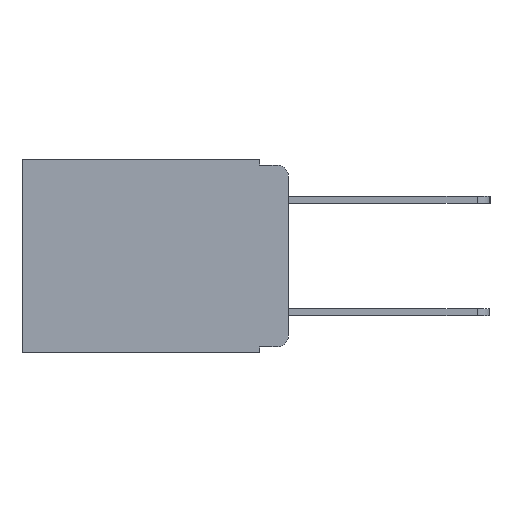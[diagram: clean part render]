
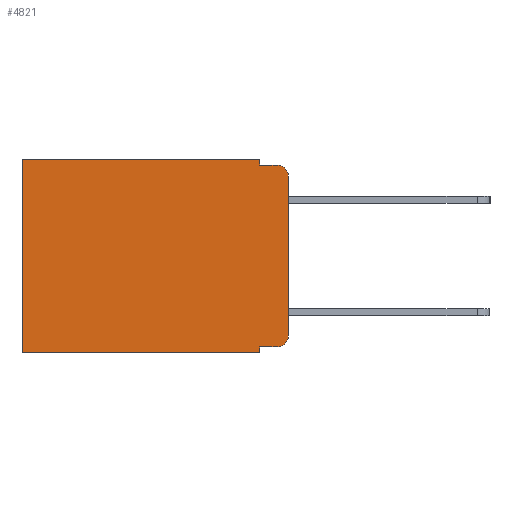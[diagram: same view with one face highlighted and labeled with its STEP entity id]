
A CAD part, left-side view. The second image highlights one B-rep face of the part: STEP entity #4821.
In plain terms, the highlighted planar face has unit normal (-1, 0, 0).
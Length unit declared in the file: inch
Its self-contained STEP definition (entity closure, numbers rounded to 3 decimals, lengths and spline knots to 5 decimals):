
#98 = DIRECTION ( 'NONE',  ( 0., 1., 0. ) ) ;
#150 = CARTESIAN_POINT ( 'NONE',  ( 0.298, 0.473, -0.343 ) ) ;
#318 = ORIENTED_EDGE ( 'NONE', *, *, #4238, .F. ) ;
#379 = VERTEX_POINT ( 'NONE', #12197 ) ;
#389 = PLANE ( 'NONE',  #3781 ) ;
#594 = DIRECTION ( 'NONE',  ( 0., 0., -1. ) ) ;
#773 = ORIENTED_EDGE ( 'NONE', *, *, #3986, .F. ) ;
#1186 = VECTOR ( 'NONE', #10258, 39.37008 ) ;
#1229 = ORIENTED_EDGE ( 'NONE', *, *, #4241, .T. ) ;
#1280 = CARTESIAN_POINT ( 'NONE',  ( 0.298, 0., -0.343 ) ) ;
#1555 = ORIENTED_EDGE ( 'NONE', *, *, #4210, .F. ) ;
#1888 = DIRECTION ( 'NONE',  ( -1., 0., 0. ) ) ;
#2179 = LINE ( 'NONE', #10203, #5570 ) ;
#2844 = DIRECTION ( 'NONE',  ( 0., 1., 0. ) ) ;
#2897 = CARTESIAN_POINT ( 'NONE',  ( 0.298, 0.051, -0.333 ) ) ;
#3305 = DIRECTION ( 'NONE',  ( 0., 0., -1. ) ) ;
#3537 = CARTESIAN_POINT ( 'NONE',  ( 0.298, 0., 0. ) ) ;
#3640 = EDGE_CURVE ( 'NONE', #8289, #14231, #14062, .T. ) ;
#3781 = AXIS2_PLACEMENT_3D ( 'NONE', #3537, #12635, #4957 ) ;
#3828 = CARTESIAN_POINT ( 'NONE',  ( 0.298, 0., -0.313 ) ) ;
#3986 = EDGE_CURVE ( 'NONE', #13887, #12372, #10531, .T. ) ;
#4166 = EDGE_CURVE ( 'NONE', #379, #12834, #6839, .T. ) ;
#4185 = EDGE_CURVE ( 'NONE', #379, #5580, #13086, .T. ) ;
#4210 = EDGE_CURVE ( 'NONE', #14830, #5580, #9556, .T. ) ;
#4213 = EDGE_CURVE ( 'NONE', #8289, #14830, #2179, .T. ) ;
#4215 = EDGE_CURVE ( 'NONE', #14231, #12372, #9168, .T. ) ;
#4238 = EDGE_CURVE ( 'NONE', #14601, #13887, #5143, .T. ) ;
#4241 = EDGE_CURVE ( 'NONE', #14601, #8076, #12006, .T. ) ;
#4269 = EDGE_CURVE ( 'NONE', #8076, #12834, #8367, .T. ) ;
#4493 = AXIS2_PLACEMENT_3D ( 'NONE', #10161, #1888, #11385 ) ;
#4821 = ADVANCED_FACE ( 'NONE', ( #11829 ), #389, .F. ) ;
#4917 = DIRECTION ( 'NONE',  ( 0., 0., -1. ) ) ;
#4957 = DIRECTION ( 'NONE',  ( 0., 0., -1. ) ) ;
#5143 = LINE ( 'NONE', #14980, #1186 ) ;
#5570 = VECTOR ( 'NONE', #4917, 39.37008 ) ;
#5580 = VERTEX_POINT ( 'NONE', #13202 ) ;
#5706 = ORIENTED_EDGE ( 'NONE', *, *, #4215, .T. ) ;
#6314 = CARTESIAN_POINT ( 'NONE',  ( 0.298, 0.051, -0.333 ) ) ;
#6353 = CARTESIAN_POINT ( 'NONE',  ( 0.298, 0.051, -0.01 ) ) ;
#6839 = LINE ( 'NONE', #10111, #9954 ) ;
#7806 = ORIENTED_EDGE ( 'NONE', *, *, #4166, .F. ) ;
#8076 = VERTEX_POINT ( 'NONE', #8678 ) ;
#8214 = ORIENTED_EDGE ( 'NONE', *, *, #4269, .T. ) ;
#8289 = VERTEX_POINT ( 'NONE', #11605 ) ;
#8367 = CIRCLE ( 'NONE', #10673, 0.02 ) ;
#8422 = ORIENTED_EDGE ( 'NONE', *, *, #4185, .T. ) ;
#8613 = ORIENTED_EDGE ( 'NONE', *, *, #4213, .F. ) ;
#8678 = CARTESIAN_POINT ( 'NONE',  ( 0.298, 0.02, -0.333 ) ) ;
#9118 = ORIENTED_EDGE ( 'NONE', *, *, #3640, .T. ) ;
#9121 = DIRECTION ( 'NONE',  ( -1., 0., 0. ) ) ;
#9168 = LINE ( 'NONE', #14935, #15105 ) ;
#9556 = LINE ( 'NONE', #11443, #12366 ) ;
#9954 = VECTOR ( 'NONE', #3305, 39.37008 ) ;
#9975 = CARTESIAN_POINT ( 'NONE',  ( 0.298, 0., 0. ) ) ;
#10111 = CARTESIAN_POINT ( 'NONE',  ( 0.298, 0., 0. ) ) ;
#10161 = CARTESIAN_POINT ( 'NONE',  ( 0.298, 0.02, -0.03 ) ) ;
#10166 = VECTOR ( 'NONE', #98, 39.37008 ) ;
#10203 = CARTESIAN_POINT ( 'NONE',  ( 0.298, 0.051, 0. ) ) ;
#10258 = DIRECTION ( 'NONE',  ( 0., 0., -1. ) ) ;
#10313 = DIRECTION ( 'NONE',  ( 0., -1., 0. ) ) ;
#10531 = LINE ( 'NONE', #1280, #16259 ) ;
#10621 = EDGE_LOOP ( 'NONE', ( #7806, #8422, #1555, #8613, #9118, #5706, #773, #318, #1229, #8214 ) ) ;
#10673 = AXIS2_PLACEMENT_3D ( 'NONE', #16092, #9121, #594 ) ;
#11385 = DIRECTION ( 'NONE',  ( 0., 0., -1. ) ) ;
#11443 = CARTESIAN_POINT ( 'NONE',  ( 0.298, 0.051, -0.01 ) ) ;
#11605 = CARTESIAN_POINT ( 'NONE',  ( 0.298, 0.051, 0. ) ) ;
#11663 = VECTOR ( 'NONE', #10313, 39.37008 ) ;
#11829 = FACE_OUTER_BOUND ( 'NONE', #10621, .T. ) ;
#12006 = LINE ( 'NONE', #6314, #11663 ) ;
#12197 = CARTESIAN_POINT ( 'NONE',  ( 0.298, 0., -0.03 ) ) ;
#12366 = VECTOR ( 'NONE', #12601, 39.37008 ) ;
#12372 = VERTEX_POINT ( 'NONE', #150 ) ;
#12601 = DIRECTION ( 'NONE',  ( 0., -1., 0. ) ) ;
#12635 = DIRECTION ( 'NONE',  ( 1., 0., 0. ) ) ;
#12834 = VERTEX_POINT ( 'NONE', #3828 ) ;
#13086 = CIRCLE ( 'NONE', #4493, 0.02 ) ;
#13202 = CARTESIAN_POINT ( 'NONE',  ( 0.298, 0.02, -0.01 ) ) ;
#13887 = VERTEX_POINT ( 'NONE', #15648 ) ;
#14062 = LINE ( 'NONE', #9975, #10166 ) ;
#14231 = VERTEX_POINT ( 'NONE', #16153 ) ;
#14601 = VERTEX_POINT ( 'NONE', #2897 ) ;
#14830 = VERTEX_POINT ( 'NONE', #6353 ) ;
#14935 = CARTESIAN_POINT ( 'NONE',  ( 0.298, 0.473, 0. ) ) ;
#14980 = CARTESIAN_POINT ( 'NONE',  ( 0.298, 0.051, 0. ) ) ;
#15105 = VECTOR ( 'NONE', #15994, 39.37008 ) ;
#15648 = CARTESIAN_POINT ( 'NONE',  ( 0.298, 0.051, -0.343 ) ) ;
#15994 = DIRECTION ( 'NONE',  ( 0., 0., -1. ) ) ;
#16092 = CARTESIAN_POINT ( 'NONE',  ( 0.298, 0.02, -0.313 ) ) ;
#16153 = CARTESIAN_POINT ( 'NONE',  ( 0.298, 0.473, 0. ) ) ;
#16259 = VECTOR ( 'NONE', #2844, 39.37008 ) ;
